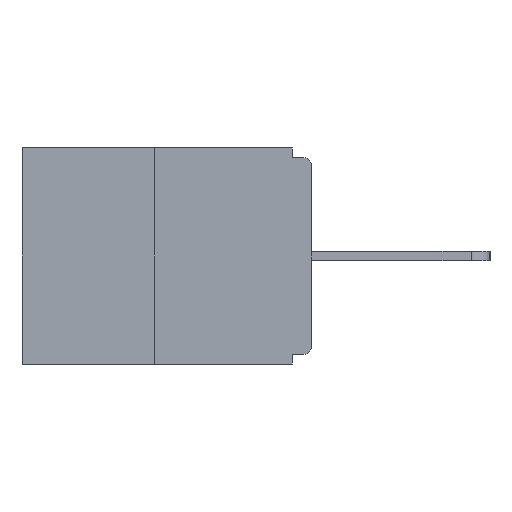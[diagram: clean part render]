
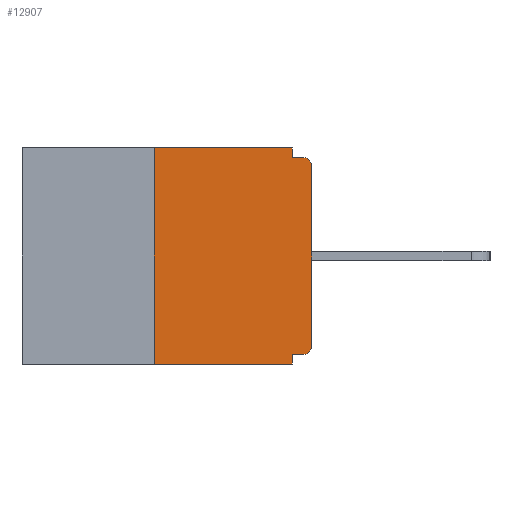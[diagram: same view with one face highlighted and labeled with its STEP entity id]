
A CAD part, left-side view. The second image highlights one B-rep face of the part: STEP entity #12907.
In plain terms, the highlighted planar face has unit normal (-1, 0, 0).
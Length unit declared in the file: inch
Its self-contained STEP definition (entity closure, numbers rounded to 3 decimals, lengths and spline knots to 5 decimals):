
#79 = ORIENTED_EDGE ( 'NONE', *, *, #11504, .T. ) ;
#94 = VERTEX_POINT ( 'NONE', #1502 ) ;
#201 = CARTESIAN_POINT ( 'NONE',  ( 0., 0.031, -0.328 ) ) ;
#431 = DIRECTION ( 'NONE',  ( 0., 0., 1. ) ) ;
#538 = AXIS2_PLACEMENT_3D ( 'NONE', #2480, #8313, #11654 ) ;
#1171 = EDGE_CURVE ( 'NONE', #94, #5127, #9905, .T. ) ;
#1374 = DIRECTION ( 'NONE',  ( 0., -1., 0. ) ) ;
#1502 = CARTESIAN_POINT ( 'NONE',  ( 0., 0., -0.313 ) ) ;
#1863 = DIRECTION ( 'NONE',  ( 0., 0., -1. ) ) ;
#1958 = EDGE_CURVE ( 'NONE', #4666, #7197, #9134, .T. ) ;
#1960 = ORIENTED_EDGE ( 'NONE', *, *, #1171, .T. ) ;
#1962 = CARTESIAN_POINT ( 'NONE',  ( 0., 0., -0.015 ) ) ;
#2349 = DIRECTION ( 'NONE',  ( 0., 0., 1. ) ) ;
#2480 = CARTESIAN_POINT ( 'NONE',  ( 0., 0.015, -0.313 ) ) ;
#2586 = EDGE_CURVE ( 'NONE', #5436, #9203, #3781, .T. ) ;
#2905 = CARTESIAN_POINT ( 'NONE',  ( 0., 0.015, -0.328 ) ) ;
#2947 = VERTEX_POINT ( 'NONE', #2905 ) ;
#3032 = ORIENTED_EDGE ( 'NONE', *, *, #1958, .T. ) ;
#3386 = VERTEX_POINT ( 'NONE', #201 ) ;
#3523 = AXIS2_PLACEMENT_3D ( 'NONE', #11599, #8395, #10514 ) ;
#3704 = VECTOR ( 'NONE', #431, 39.37008 ) ;
#3781 = LINE ( 'NONE', #12598, #12581 ) ;
#3859 = PLANE ( 'NONE',  #11456 ) ;
#3867 = ORIENTED_EDGE ( 'NONE', *, *, #2586, .F. ) ;
#4018 = DIRECTION ( 'NONE',  ( 0., -1., 0. ) ) ;
#4062 = ORIENTED_EDGE ( 'NONE', *, *, #4067, .F. ) ;
#4067 = EDGE_CURVE ( 'NONE', #2947, #3386, #12647, .T. ) ;
#4070 = FACE_OUTER_BOUND ( 'NONE', #6637, .T. ) ;
#4158 = VECTOR ( 'NONE', #8627, 39.37008 ) ;
#4223 = CARTESIAN_POINT ( 'NONE',  ( 0., 0.25, -0.343 ) ) ;
#4598 = CARTESIAN_POINT ( 'NONE',  ( 0., 0., -0.03 ) ) ;
#4657 = VECTOR ( 'NONE', #12521, 39.37008 ) ;
#4666 = VERTEX_POINT ( 'NONE', #4223 ) ;
#4815 = ORIENTED_EDGE ( 'NONE', *, *, #6186, .F. ) ;
#4863 = CIRCLE ( 'NONE', #538, 0.015 ) ;
#5127 = VERTEX_POINT ( 'NONE', #4598 ) ;
#5436 = VERTEX_POINT ( 'NONE', #13987 ) ;
#5547 = CARTESIAN_POINT ( 'NONE',  ( 0., 0.031, -0.343 ) ) ;
#5620 = ORIENTED_EDGE ( 'NONE', *, *, #6137, .F. ) ;
#5926 = VERTEX_POINT ( 'NONE', #12271 ) ;
#6137 = EDGE_CURVE ( 'NONE', #4666, #5436, #10189, .T. ) ;
#6186 = EDGE_CURVE ( 'NONE', #3386, #7197, #14025, .T. ) ;
#6637 = EDGE_LOOP ( 'NONE', ( #3867, #5620, #3032, #4815, #4062, #12848, #1960, #79, #7370, #8647 ) ) ;
#6856 = CARTESIAN_POINT ( 'NONE',  ( 0., 0.46, -0.343 ) ) ;
#6861 = VECTOR ( 'NONE', #12506, 39.37008 ) ;
#6977 = LINE ( 'NONE', #9173, #4657 ) ;
#7197 = VERTEX_POINT ( 'NONE', #5547 ) ;
#7318 = EDGE_CURVE ( 'NONE', #2947, #94, #4863, .T. ) ;
#7370 = ORIENTED_EDGE ( 'NONE', *, *, #7801, .F. ) ;
#7801 = EDGE_CURVE ( 'NONE', #5926, #8696, #9568, .T. ) ;
#7922 = VECTOR ( 'NONE', #2349, 39.37008 ) ;
#8076 = CARTESIAN_POINT ( 'NONE',  ( 0., 0.031, 0. ) ) ;
#8313 = DIRECTION ( 'NONE',  ( -1., 0., 0. ) ) ;
#8395 = DIRECTION ( 'NONE',  ( -1., 0., 0. ) ) ;
#8621 = CARTESIAN_POINT ( 'NONE',  ( 0., 0.015, -0.015 ) ) ;
#8627 = DIRECTION ( 'NONE',  ( 0., 0., -1. ) ) ;
#8647 = ORIENTED_EDGE ( 'NONE', *, *, #13222, .F. ) ;
#8693 = CARTESIAN_POINT ( 'NONE',  ( 0., 0.031, -0.343 ) ) ;
#8696 = VERTEX_POINT ( 'NONE', #8621 ) ;
#9115 = CARTESIAN_POINT ( 'NONE',  ( 0., 0., 0. ) ) ;
#9134 = LINE ( 'NONE', #6856, #12321 ) ;
#9173 = CARTESIAN_POINT ( 'NONE',  ( 0., 0.031, 0. ) ) ;
#9203 = VERTEX_POINT ( 'NONE', #8076 ) ;
#9434 = CARTESIAN_POINT ( 'NONE',  ( 0., 0., -0.328 ) ) ;
#9549 = DIRECTION ( 'NONE',  ( 1., 0., 0. ) ) ;
#9568 = LINE ( 'NONE', #1962, #11697 ) ;
#9905 = LINE ( 'NONE', #9115, #7922 ) ;
#10189 = LINE ( 'NONE', #10247, #3704 ) ;
#10247 = CARTESIAN_POINT ( 'NONE',  ( 0., 0.25, 0. ) ) ;
#10514 = DIRECTION ( 'NONE',  ( 0., 0., -1. ) ) ;
#10571 = CIRCLE ( 'NONE', #3523, 0.015 ) ;
#11456 = AXIS2_PLACEMENT_3D ( 'NONE', #12692, #9549, #1863 ) ;
#11504 = EDGE_CURVE ( 'NONE', #5127, #8696, #10571, .T. ) ;
#11599 = CARTESIAN_POINT ( 'NONE',  ( 0., 0.015, -0.03 ) ) ;
#11654 = DIRECTION ( 'NONE',  ( 0., 0., -1. ) ) ;
#11697 = VECTOR ( 'NONE', #4018, 39.37008 ) ;
#12271 = CARTESIAN_POINT ( 'NONE',  ( 0., 0.031, -0.015 ) ) ;
#12321 = VECTOR ( 'NONE', #1374, 39.37008 ) ;
#12506 = DIRECTION ( 'NONE',  ( 0., 1., 0. ) ) ;
#12521 = DIRECTION ( 'NONE',  ( 0., 0., -1. ) ) ;
#12581 = VECTOR ( 'NONE', #13591, 39.37008 ) ;
#12598 = CARTESIAN_POINT ( 'NONE',  ( 0., 0.46, 0. ) ) ;
#12647 = LINE ( 'NONE', #9434, #6861 ) ;
#12692 = CARTESIAN_POINT ( 'NONE',  ( 0., 0.46, 0. ) ) ;
#12848 = ORIENTED_EDGE ( 'NONE', *, *, #7318, .T. ) ;
#12907 = ADVANCED_FACE ( 'NONE', ( #4070 ), #3859, .F. ) ;
#13222 = EDGE_CURVE ( 'NONE', #9203, #5926, #6977, .T. ) ;
#13591 = DIRECTION ( 'NONE',  ( 0., -1., 0. ) ) ;
#13987 = CARTESIAN_POINT ( 'NONE',  ( 0., 0.25, 0. ) ) ;
#14025 = LINE ( 'NONE', #8693, #4158 ) ;
